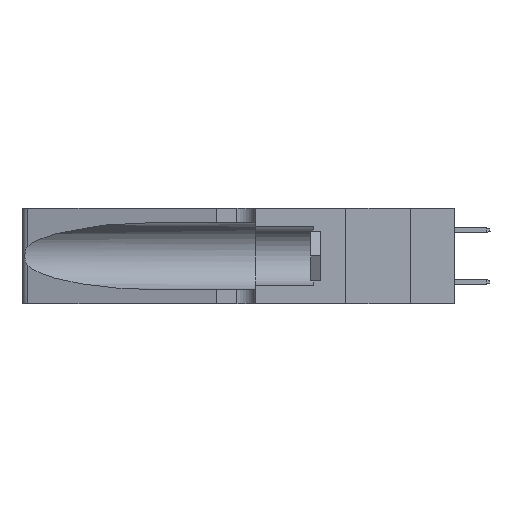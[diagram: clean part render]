
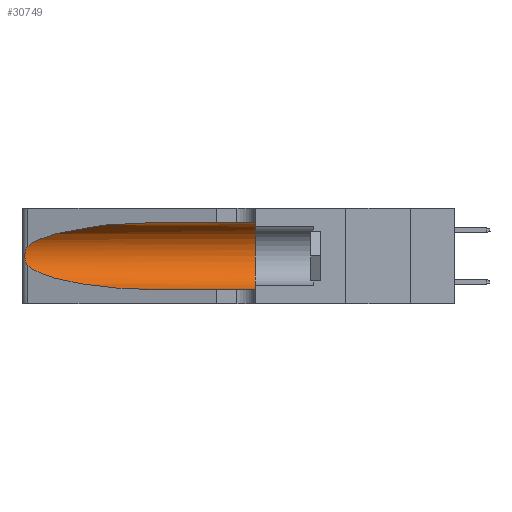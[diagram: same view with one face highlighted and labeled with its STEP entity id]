
A CAD part, left-side view. The second image highlights one B-rep face of the part: STEP entity #30749.
In plain terms, the highlighted cylindrical face has radius 3.308 mm (diameter 6.617 mm), a partial arc.
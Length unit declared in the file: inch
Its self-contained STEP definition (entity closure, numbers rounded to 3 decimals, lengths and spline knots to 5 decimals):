
#263 = CARTESIAN_POINT ( 'NONE',  ( 0.25856, 1.23593, 0.16098 ) ) ;
#1032 = LINE ( 'NONE', #28714, #28711 ) ;
#1127 = CARTESIAN_POINT ( 'NONE',  ( 0.1305, 1.61858, 0.05475 ) ) ;
#1316 = CARTESIAN_POINT ( 'NONE',  ( 0.1305, 0.72297, 0.05475 ) ) ;
#1789 = EDGE_CURVE ( 'NONE', #6092, #20297, #18628, .T. ) ;
#1883 = CARTESIAN_POINT ( 'NONE',  ( 0.1305, 0.35, 0.31525 ) ) ;
#4563 = ORIENTED_EDGE ( 'NONE', *, *, #22264, .T. ) ;
#6092 = VERTEX_POINT ( 'NONE', #35128 ) ;
#6335 = CARTESIAN_POINT ( 'NONE',  ( 0.25789, 1.23486, 0.15765 ) ) ;
#6998 = DIRECTION ( 'NONE',  ( 0., -1., 0. ) ) ;
#7494 = ORIENTED_EDGE ( 'NONE', *, *, #1789, .T. ) ;
#8679 = AXIS2_PLACEMENT_3D ( 'NONE', #14173, #26539, #38862 ) ;
#9564 = CARTESIAN_POINT ( 'NONE',  ( 0.25787, 1.23484, 0.2124 ) ) ;
#9851 = DIRECTION ( 'NONE',  ( 0., 0., -1. ) ) ;
#10046 = CARTESIAN_POINT ( 'NONE',  ( 0.1305, 1.61858, 0.185 ) ) ;
#10306 = DIRECTION ( 'NONE',  ( 0., -1., 0. ) ) ;
#10322 = B_SPLINE_CURVE_WITH_KNOTS ( 'NONE', 3,
 ( #12579, #24544, #28341, #9564, #15406, #21878, #15621, #39843, #34211, #263, #6335, #27771, #18635, #25346 ),
 .UNSPECIFIED., .F., .F.,
 ( 4, 2, 2, 2, 2, 2, 4 ),
 ( 0., 0.00027, 0.00053, 0.00107, 0.0016, 0.00187, 0.00214 ),
 .UNSPECIFIED. ) ;
#11599 = EDGE_CURVE ( 'NONE', #20297, #32475, #10322, .T. ) ;
#12020 = CARTESIAN_POINT ( 'NONE',  ( 0.25487, 1.22718, 0.22369 ) ) ;
#12387 = EDGE_CURVE ( 'NONE', #19690, #38615, #17692, .T. ) ;
#12579 = CARTESIAN_POINT ( 'NONE',  ( 0.25487, 1.22718, 0.22369 ) ) ;
#14173 = CARTESIAN_POINT ( 'NONE',  ( 0.1305, 0.35, 0.185 ) ) ;
#15406 = CARTESIAN_POINT ( 'NONE',  ( 0.25854, 1.2359, 0.20912 ) ) ;
#15576 = EDGE_LOOP ( 'NONE', ( #7494, #19939, #17314, #4563, #19813, #21980 ) ) ;
#15621 = CARTESIAN_POINT ( 'NONE',  ( 0.26075, 1.23896, 0.19203 ) ) ;
#16121 = CARTESIAN_POINT ( 'NONE',  ( 0.18966, 0.96281, 0.05475 ) ) ;
#16216 = EDGE_CURVE ( 'NONE', #6092, #19690, #1032, .T. ) ;
#17314 = ORIENTED_EDGE ( 'NONE', *, *, #36622, .T. ) ;
#17692 = CIRCLE ( 'NONE', #8679, 0.13025 ) ;
#18105 = CARTESIAN_POINT ( 'NONE',  ( 0.1305, 0.35, 0.05475 ) ) ;
#18628 =( BOUNDED_CURVE ( )  B_SPLINE_CURVE ( 3, ( #35818, #29991, #23716, #20276 ),
 .UNSPECIFIED., .F., .T. ) 
 B_SPLINE_CURVE_WITH_KNOTS ( ( 4, 4 ),
 ( 1.5708, 2.84003 ),
 .UNSPECIFIED. ) 
 CURVE ( )  GEOMETRIC_REPRESENTATION_ITEM ( )  RATIONAL_B_SPLINE_CURVE ( ( 1., 0.87, 0.87, 1. ) ) 
 REPRESENTATION_ITEM ( '' )  );
#18635 = CARTESIAN_POINT ( 'NONE',  ( 0.25555, 1.22993, 0.14849 ) ) ;
#19394 = VECTOR ( 'NONE', #6998, 39.37008 ) ;
#19543 = DIRECTION ( 'NONE',  ( 0., -1., 0. ) ) ;
#19690 = VERTEX_POINT ( 'NONE', #1883 ) ;
#19813 = ORIENTED_EDGE ( 'NONE', *, *, #12387, .F. ) ;
#19939 = ORIENTED_EDGE ( 'NONE', *, *, #11599, .T. ) ;
#20276 = CARTESIAN_POINT ( 'NONE',  ( 0.25487, 1.22718, 0.22369 ) ) ;
#20297 = VERTEX_POINT ( 'NONE', #12020 ) ;
#21878 = CARTESIAN_POINT ( 'NONE',  ( 0.26018, 1.23835, 0.19895 ) ) ;
#21980 = ORIENTED_EDGE ( 'NONE', *, *, #16216, .F. ) ;
#22264 = EDGE_CURVE ( 'NONE', #22265, #38615, #38284, .T. ) ;
#22265 = VERTEX_POINT ( 'NONE', #1316 ) ;
#22365 = CYLINDRICAL_SURFACE ( 'NONE', #39321, 0.13025 ) ;
#23716 = CARTESIAN_POINT ( 'NONE',  ( 0.2373, 1.15595, 0.28018 ) ) ;
#24544 = CARTESIAN_POINT ( 'NONE',  ( 0.25555, 1.22994, 0.2215 ) ) ;
#25069 = CARTESIAN_POINT ( 'NONE',  ( 0.2373, 1.15595, 0.08982 ) ) ;
#25346 = CARTESIAN_POINT ( 'NONE',  ( 0.25487, 1.22718, 0.14631 ) ) ;
#26539 = DIRECTION ( 'NONE',  ( 0., 1., 0. ) ) ;
#27771 = CARTESIAN_POINT ( 'NONE',  ( 0.25639, 1.23186, 0.15144 ) ) ;
#28341 = CARTESIAN_POINT ( 'NONE',  ( 0.25639, 1.23184, 0.21858 ) ) ;
#28711 = VECTOR ( 'NONE', #10306, 39.37008 ) ;
#28714 = CARTESIAN_POINT ( 'NONE',  ( 0.1305, 1.61858, 0.31525 ) ) ;
#28830 = FACE_OUTER_BOUND ( 'NONE', #15576, .T. ) ;
#29991 = CARTESIAN_POINT ( 'NONE',  ( 0.18966, 0.96281, 0.31525 ) ) ;
#30749 = ADVANCED_FACE ( 'NONE', ( #28830 ), #22365, .F. ) ;
#31324 = CARTESIAN_POINT ( 'NONE',  ( 0.1305, 0.72297, 0.05475 ) ) ;
#32475 = VERTEX_POINT ( 'NONE', #34194 ) ;
#34194 = CARTESIAN_POINT ( 'NONE',  ( 0.25487, 1.22718, 0.14631 ) ) ;
#34211 = CARTESIAN_POINT ( 'NONE',  ( 0.26017, 1.23833, 0.17102 ) ) ;
#35128 = CARTESIAN_POINT ( 'NONE',  ( 0.1305, 0.72297, 0.31525 ) ) ;
#35818 = CARTESIAN_POINT ( 'NONE',  ( 0.1305, 0.72297, 0.31525 ) ) ;
#36622 = EDGE_CURVE ( 'NONE', #32475, #22265, #37833, .T. ) ;
#37755 = CARTESIAN_POINT ( 'NONE',  ( 0.25487, 1.22718, 0.14631 ) ) ;
#37833 =( BOUNDED_CURVE ( )  B_SPLINE_CURVE ( 3, ( #37755, #25069, #16121, #31324 ),
 .UNSPECIFIED., .F., .T. ) 
 B_SPLINE_CURVE_WITH_KNOTS ( ( 4, 4 ),
 ( 3.44316, 4.71239 ),
 .UNSPECIFIED. ) 
 CURVE ( )  GEOMETRIC_REPRESENTATION_ITEM ( )  RATIONAL_B_SPLINE_CURVE ( ( 1., 0.87, 0.87, 1. ) ) 
 REPRESENTATION_ITEM ( '' )  );
#38284 = LINE ( 'NONE', #1127, #19394 ) ;
#38615 = VERTEX_POINT ( 'NONE', #18105 ) ;
#38862 = DIRECTION ( 'NONE',  ( 0., 0., 1. ) ) ;
#39321 = AXIS2_PLACEMENT_3D ( 'NONE', #10046, #19543, #9851 ) ;
#39843 = CARTESIAN_POINT ( 'NONE',  ( 0.26075, 1.23896, 0.178 ) ) ;
